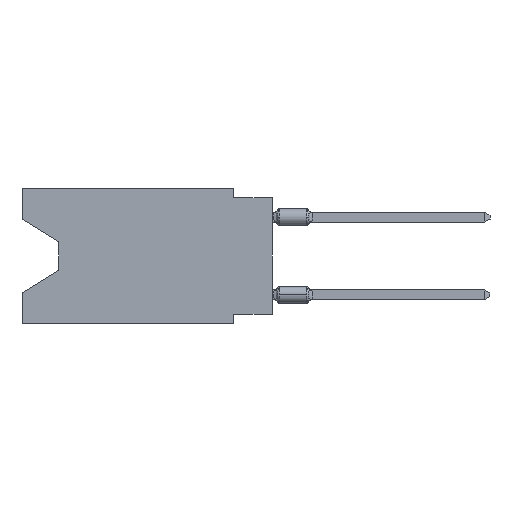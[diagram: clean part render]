
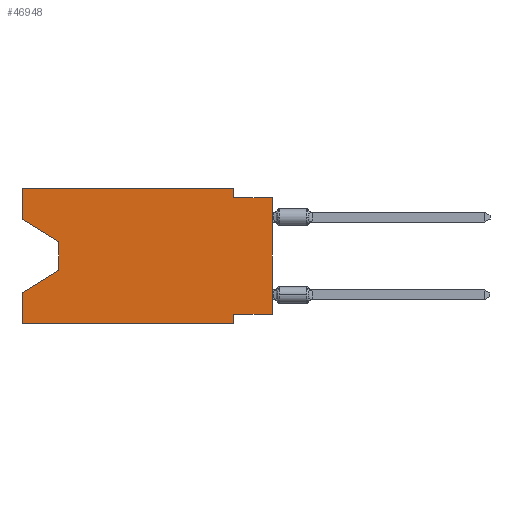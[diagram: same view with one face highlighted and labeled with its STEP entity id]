
A CAD part, left-side view. The second image highlights one B-rep face of the part: STEP entity #46948.
In plain terms, the highlighted planar face has unit normal (-1, 0, 0).
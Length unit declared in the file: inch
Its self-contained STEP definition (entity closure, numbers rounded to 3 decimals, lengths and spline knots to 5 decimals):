
#233 = CARTESIAN_POINT ( 'NONE',  ( 0., 0., -0.025 ) ) ;
#1263 = DIRECTION ( 'NONE',  ( 0., -1., 0. ) ) ;
#1417 = PLANE ( 'NONE',  #43369 ) ;
#1555 = EDGE_CURVE ( 'NONE', #6994, #17395, #33314, .T. ) ;
#1926 = DIRECTION ( 'NONE',  ( 0., 0., -1. ) ) ;
#2172 = EDGE_CURVE ( 'NONE', #28706, #12704, #9598, .T. ) ;
#2408 = VECTOR ( 'NONE', #46330, 39.37008 ) ;
#3475 = VERTEX_POINT ( 'NONE', #40874 ) ;
#3812 = CARTESIAN_POINT ( 'NONE',  ( 0., 0.1, -0.35 ) ) ;
#6620 = VECTOR ( 'NONE', #1263, 39.37008 ) ;
#6994 = VERTEX_POINT ( 'NONE', #45271 ) ;
#7036 = EDGE_LOOP ( 'NONE', ( #45988, #33754, #50548, #11595, #14277, #26359, #8881, #16069, #25501, #11747, #30607, #11421 ) ) ;
#7173 = VECTOR ( 'NONE', #25115, 39.37008 ) ;
#8724 = LINE ( 'NONE', #45784, #2408 ) ;
#8881 = ORIENTED_EDGE ( 'NONE', *, *, #50488, .F. ) ;
#9525 = DIRECTION ( 'NONE',  ( 0., 0., -1. ) ) ;
#9598 = LINE ( 'NONE', #18172, #6620 ) ;
#10055 = CARTESIAN_POINT ( 'NONE',  ( 0., 0.645, 0. ) ) ;
#10081 = VECTOR ( 'NONE', #41644, 39.37008 ) ;
#10086 = CARTESIAN_POINT ( 'NONE',  ( 0., 0.645, 0. ) ) ;
#11421 = ORIENTED_EDGE ( 'NONE', *, *, #52942, .F. ) ;
#11595 = ORIENTED_EDGE ( 'NONE', *, *, #34985, .F. ) ;
#11747 = ORIENTED_EDGE ( 'NONE', *, *, #36686, .F. ) ;
#12212 = LINE ( 'NONE', #22387, #36617 ) ;
#12332 = VECTOR ( 'NONE', #50009, 39.37008 ) ;
#12704 = VERTEX_POINT ( 'NONE', #233 ) ;
#13308 = DIRECTION ( 'NONE',  ( 0., -1., 0. ) ) ;
#13482 = LINE ( 'NONE', #46255, #19371 ) ;
#14022 = CARTESIAN_POINT ( 'NONE',  ( 0., 0.645, 0. ) ) ;
#14277 = ORIENTED_EDGE ( 'NONE', *, *, #49590, .T. ) ;
#14364 = VERTEX_POINT ( 'NONE', #35197 ) ;
#15310 = VERTEX_POINT ( 'NONE', #3812 ) ;
#16069 = ORIENTED_EDGE ( 'NONE', *, *, #37408, .T. ) ;
#16679 = CARTESIAN_POINT ( 'NONE',  ( 0., 0.55, -0.212 ) ) ;
#17395 = VERTEX_POINT ( 'NONE', #46764 ) ;
#18072 = DIRECTION ( 'NONE',  ( 1., 0., 0. ) ) ;
#18172 = CARTESIAN_POINT ( 'NONE',  ( 0., 0., -0.025 ) ) ;
#19371 = VECTOR ( 'NONE', #38180, 39.37008 ) ;
#20323 = CARTESIAN_POINT ( 'NONE',  ( 0., 0., 0. ) ) ;
#22387 = CARTESIAN_POINT ( 'NONE',  ( 0., 0.1, 0. ) ) ;
#23306 = VERTEX_POINT ( 'NONE', #25672 ) ;
#24276 = DIRECTION ( 'NONE',  ( 0., 1., 0. ) ) ;
#24759 = VECTOR ( 'NONE', #24276, 39.37008 ) ;
#24791 = CARTESIAN_POINT ( 'NONE',  ( 0., 0.1, -0.025 ) ) ;
#25115 = DIRECTION ( 'NONE',  ( 0., 0., 1. ) ) ;
#25501 = ORIENTED_EDGE ( 'NONE', *, *, #2172, .F. ) ;
#25511 = CARTESIAN_POINT ( 'NONE',  ( 0., 0.55, -0.138 ) ) ;
#25587 = FACE_OUTER_BOUND ( 'NONE', #7036, .T. ) ;
#25672 = CARTESIAN_POINT ( 'NONE',  ( 0., 0., -0.325 ) ) ;
#25796 = CARTESIAN_POINT ( 'NONE',  ( 0., 0.645, 0. ) ) ;
#25938 = LINE ( 'NONE', #42335, #34212 ) ;
#26359 = ORIENTED_EDGE ( 'NONE', *, *, #50183, .F. ) ;
#28628 = LINE ( 'NONE', #20323, #7173 ) ;
#28706 = VERTEX_POINT ( 'NONE', #24791 ) ;
#28755 = LINE ( 'NONE', #25511, #10081 ) ;
#29781 = VERTEX_POINT ( 'NONE', #40131 ) ;
#30518 = DIRECTION ( 'NONE',  ( 0., 0., -1. ) ) ;
#30607 = ORIENTED_EDGE ( 'NONE', *, *, #52031, .F. ) ;
#31534 = VECTOR ( 'NONE', #33031, 39.37008 ) ;
#33031 = DIRECTION ( 'NONE',  ( 0., -0.855, -0.519 ) ) ;
#33314 = LINE ( 'NONE', #41362, #31534 ) ;
#33604 = LINE ( 'NONE', #25796, #12332 ) ;
#33754 = ORIENTED_EDGE ( 'NONE', *, *, #43788, .T. ) ;
#34212 = VECTOR ( 'NONE', #30518, 39.37008 ) ;
#34985 = EDGE_CURVE ( 'NONE', #45228, #29781, #13482, .T. ) ;
#35197 = CARTESIAN_POINT ( 'NONE',  ( 0., 0.1, 0. ) ) ;
#35669 = CARTESIAN_POINT ( 'NONE',  ( 0., 0.1, -0.325 ) ) ;
#35687 = VERTEX_POINT ( 'NONE', #10055 ) ;
#36032 = LINE ( 'NONE', #16679, #48628 ) ;
#36617 = VECTOR ( 'NONE', #9525, 39.37008 ) ;
#36686 = EDGE_CURVE ( 'NONE', #14364, #28706, #12212, .T. ) ;
#36913 = LINE ( 'NONE', #40957, #24759 ) ;
#37408 = EDGE_CURVE ( 'NONE', #23306, #12704, #28628, .T. ) ;
#38007 = LINE ( 'NONE', #10086, #50863 ) ;
#38180 = DIRECTION ( 'NONE',  ( 0., 0., 1. ) ) ;
#40131 = CARTESIAN_POINT ( 'NONE',  ( 0., 0.645, -0.26975 ) ) ;
#40874 = CARTESIAN_POINT ( 'NONE',  ( 0., 0.55, -0.212 ) ) ;
#40957 = CARTESIAN_POINT ( 'NONE',  ( 0., 0., -0.325 ) ) ;
#41253 = EDGE_CURVE ( 'NONE', #3475, #29781, #36032, .T. ) ;
#41362 = CARTESIAN_POINT ( 'NONE',  ( 0., 0.645, -0.08025 ) ) ;
#41644 = DIRECTION ( 'NONE',  ( 0., 0., -1. ) ) ;
#42335 = CARTESIAN_POINT ( 'NONE',  ( 0., 0.1, -0.35 ) ) ;
#43369 = AXIS2_PLACEMENT_3D ( 'NONE', #14022, #18072, #1926 ) ;
#43788 = EDGE_CURVE ( 'NONE', #17395, #3475, #28755, .T. ) ;
#44370 = DIRECTION ( 'NONE',  ( 0., 0.855, -0.519 ) ) ;
#45228 = VERTEX_POINT ( 'NONE', #45467 ) ;
#45271 = CARTESIAN_POINT ( 'NONE',  ( 0., 0.645, -0.08025 ) ) ;
#45467 = CARTESIAN_POINT ( 'NONE',  ( 0., 0.645, -0.35 ) ) ;
#45784 = CARTESIAN_POINT ( 'NONE',  ( 0., 0.645, -0.35 ) ) ;
#45988 = ORIENTED_EDGE ( 'NONE', *, *, #1555, .T. ) ;
#46255 = CARTESIAN_POINT ( 'NONE',  ( 0., 0.645, 0. ) ) ;
#46330 = DIRECTION ( 'NONE',  ( 0., -1., 0. ) ) ;
#46764 = CARTESIAN_POINT ( 'NONE',  ( 0., 0.55, -0.138 ) ) ;
#46948 = ADVANCED_FACE ( 'NONE', ( #25587 ), #1417, .F. ) ;
#48628 = VECTOR ( 'NONE', #44370, 39.37008 ) ;
#49590 = EDGE_CURVE ( 'NONE', #45228, #15310, #8724, .T. ) ;
#50009 = DIRECTION ( 'NONE',  ( 0., 0., 1. ) ) ;
#50183 = EDGE_CURVE ( 'NONE', #51674, #15310, #25938, .T. ) ;
#50488 = EDGE_CURVE ( 'NONE', #23306, #51674, #36913, .T. ) ;
#50548 = ORIENTED_EDGE ( 'NONE', *, *, #41253, .T. ) ;
#50863 = VECTOR ( 'NONE', #13308, 39.37008 ) ;
#51674 = VERTEX_POINT ( 'NONE', #35669 ) ;
#52031 = EDGE_CURVE ( 'NONE', #35687, #14364, #38007, .T. ) ;
#52942 = EDGE_CURVE ( 'NONE', #6994, #35687, #33604, .T. ) ;
